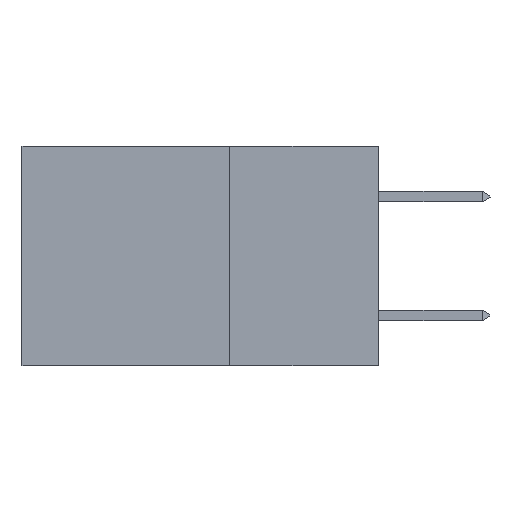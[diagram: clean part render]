
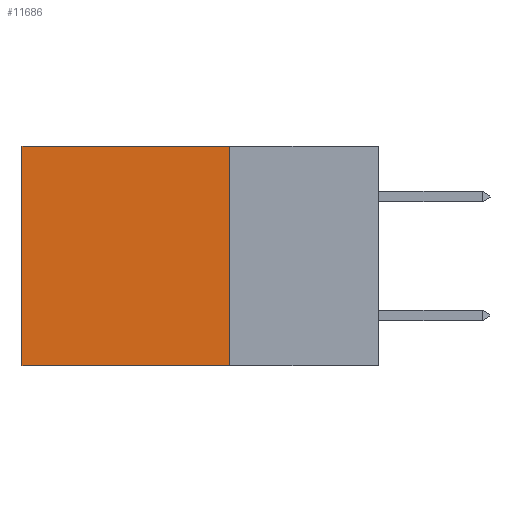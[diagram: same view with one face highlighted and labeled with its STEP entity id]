
A CAD part, left-side view. The second image highlights one B-rep face of the part: STEP entity #11686.
In plain terms, the highlighted planar face has unit normal (-1, 0, 0).
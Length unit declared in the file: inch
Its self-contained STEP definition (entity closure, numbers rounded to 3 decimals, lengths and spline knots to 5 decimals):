
#87 = EDGE_CURVE ( 'NONE', #14925, #283, #1990, .T. ) ;
#283 = VERTEX_POINT ( 'NONE', #3943 ) ;
#321 = CARTESIAN_POINT ( 'NONE',  ( 0.298, 0.6, 0. ) ) ;
#629 = EDGE_LOOP ( 'NONE', ( #3291, #11160, #15323, #13984 ) ) ;
#846 = DIRECTION ( 'NONE',  ( 0., 0., -1. ) ) ;
#937 = VECTOR ( 'NONE', #12656, 39.37008 ) ;
#1609 = DIRECTION ( 'NONE',  ( 0., 0., -1. ) ) ;
#1693 = VECTOR ( 'NONE', #5202, 39.37008 ) ;
#1706 = EDGE_CURVE ( 'NONE', #14058, #283, #11157, .T. ) ;
#1990 = LINE ( 'NONE', #321, #9788 ) ;
#2093 = LINE ( 'NONE', #9027, #1693 ) ;
#2348 = CARTESIAN_POINT ( 'NONE',  ( 0.298, 0.25, -0.37 ) ) ;
#3066 = AXIS2_PLACEMENT_3D ( 'NONE', #16114, #11042, #846 ) ;
#3291 = ORIENTED_EDGE ( 'NONE', *, *, #87, .T. ) ;
#3943 = CARTESIAN_POINT ( 'NONE',  ( 0.298, 0.6, -0.37 ) ) ;
#4891 = VERTEX_POINT ( 'NONE', #5626 ) ;
#5202 = DIRECTION ( 'NONE',  ( 0., 1., 0. ) ) ;
#5572 = EDGE_CURVE ( 'NONE', #4891, #14925, #2093, .T. ) ;
#5626 = CARTESIAN_POINT ( 'NONE',  ( 0.298, 0.25, 0. ) ) ;
#7927 = FACE_OUTER_BOUND ( 'NONE', #629, .T. ) ;
#8529 = PLANE ( 'NONE',  #3066 ) ;
#9027 = CARTESIAN_POINT ( 'NONE',  ( 0.298, 0.25, 0. ) ) ;
#9423 = VECTOR ( 'NONE', #11713, 39.37008 ) ;
#9788 = VECTOR ( 'NONE', #1609, 39.37008 ) ;
#10042 = LINE ( 'NONE', #12997, #9423 ) ;
#11042 = DIRECTION ( 'NONE',  ( 1., 0., 0. ) ) ;
#11157 = LINE ( 'NONE', #11373, #937 ) ;
#11160 = ORIENTED_EDGE ( 'NONE', *, *, #1706, .F. ) ;
#11373 = CARTESIAN_POINT ( 'NONE',  ( 0.298, 0.25, -0.37 ) ) ;
#11686 = ADVANCED_FACE ( 'NONE', ( #7927 ), #8529, .F. ) ;
#11713 = DIRECTION ( 'NONE',  ( 0., 0., -1. ) ) ;
#12656 = DIRECTION ( 'NONE',  ( 0., 1., 0. ) ) ;
#12997 = CARTESIAN_POINT ( 'NONE',  ( 0.298, 0.25, 0. ) ) ;
#13984 = ORIENTED_EDGE ( 'NONE', *, *, #5572, .T. ) ;
#14058 = VERTEX_POINT ( 'NONE', #2348 ) ;
#14401 = EDGE_CURVE ( 'NONE', #4891, #14058, #10042, .T. ) ;
#14925 = VERTEX_POINT ( 'NONE', #15112 ) ;
#15112 = CARTESIAN_POINT ( 'NONE',  ( 0.298, 0.6, 0. ) ) ;
#15323 = ORIENTED_EDGE ( 'NONE', *, *, #14401, .F. ) ;
#16114 = CARTESIAN_POINT ( 'NONE',  ( 0.298, 0.25, 0. ) ) ;
